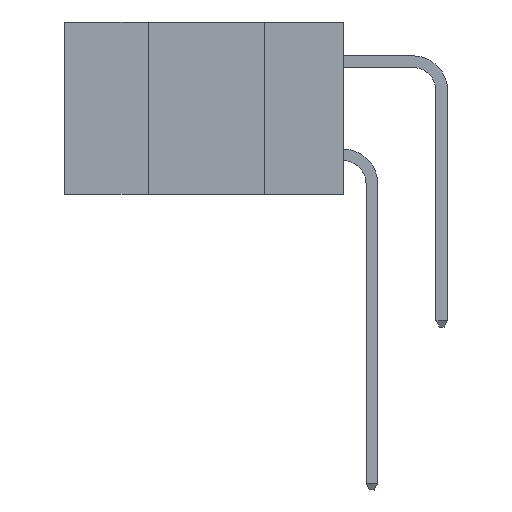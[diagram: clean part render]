
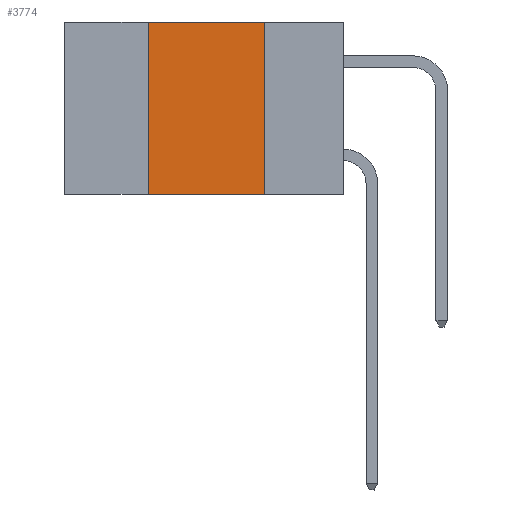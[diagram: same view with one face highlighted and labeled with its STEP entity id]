
A CAD part, left-side view. The second image highlights one B-rep face of the part: STEP entity #3774.
In plain terms, the highlighted planar face has unit normal (-1, 0, 0).
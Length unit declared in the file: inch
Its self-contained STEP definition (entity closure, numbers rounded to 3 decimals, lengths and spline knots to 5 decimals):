
#669 = ORIENTED_EDGE ( 'NONE', *, *, #6722, .T. ) ;
#713 = FACE_OUTER_BOUND ( 'NONE', #1780, .T. ) ;
#848 = CARTESIAN_POINT ( 'NONE',  ( 0., 0.42, 0. ) ) ;
#1388 = DIRECTION ( 'NONE',  ( 0., 0., -1. ) ) ;
#1756 = DIRECTION ( 'NONE',  ( 0., -1., 0. ) ) ;
#1780 = EDGE_LOOP ( 'NONE', ( #10727, #11275, #1974, #669 ) ) ;
#1974 = ORIENTED_EDGE ( 'NONE', *, *, #6973, .F. ) ;
#2211 = VERTEX_POINT ( 'NONE', #6532 ) ;
#2814 = DIRECTION ( 'NONE',  ( 1., 0., 0. ) ) ;
#3587 = AXIS2_PLACEMENT_3D ( 'NONE', #4600, #2814, #1388 ) ;
#3748 = CARTESIAN_POINT ( 'NONE',  ( 0., 0.42, -0.37 ) ) ;
#3774 = ADVANCED_FACE ( 'NONE', ( #713 ), #9079, .F. ) ;
#4600 = CARTESIAN_POINT ( 'NONE',  ( 0., 0.6, 0. ) ) ;
#4678 = CARTESIAN_POINT ( 'NONE',  ( 0., 0.6, 0. ) ) ;
#5889 = CARTESIAN_POINT ( 'NONE',  ( 0., 0.17, -0.37 ) ) ;
#5912 = VECTOR ( 'NONE', #1756, 39.37008 ) ;
#6346 = CARTESIAN_POINT ( 'NONE',  ( 0., 0.6, -0.37 ) ) ;
#6445 = VECTOR ( 'NONE', #9263, 39.37008 ) ;
#6532 = CARTESIAN_POINT ( 'NONE',  ( 0., 0.17, 0. ) ) ;
#6722 = EDGE_CURVE ( 'NONE', #8249, #11709, #11407, .T. ) ;
#6894 = LINE ( 'NONE', #4678, #6445 ) ;
#6973 = EDGE_CURVE ( 'NONE', #8249, #10506, #10831, .T. ) ;
#7071 = EDGE_CURVE ( 'NONE', #2211, #11709, #10114, .T. ) ;
#7792 = VECTOR ( 'NONE', #7807, 39.37008 ) ;
#7807 = DIRECTION ( 'NONE',  ( 0., 0., 1. ) ) ;
#8249 = VERTEX_POINT ( 'NONE', #3748 ) ;
#8517 = EDGE_CURVE ( 'NONE', #10506, #2211, #6894, .T. ) ;
#9079 = PLANE ( 'NONE',  #3587 ) ;
#9263 = DIRECTION ( 'NONE',  ( 0., -1., 0. ) ) ;
#9363 = VECTOR ( 'NONE', #10874, 39.37008 ) ;
#9485 = CARTESIAN_POINT ( 'NONE',  ( 0., 0.42, 0. ) ) ;
#9984 = CARTESIAN_POINT ( 'NONE',  ( 0., 0.17, 0. ) ) ;
#10114 = LINE ( 'NONE', #9984, #9363 ) ;
#10506 = VERTEX_POINT ( 'NONE', #848 ) ;
#10727 = ORIENTED_EDGE ( 'NONE', *, *, #7071, .F. ) ;
#10831 = LINE ( 'NONE', #9485, #7792 ) ;
#10874 = DIRECTION ( 'NONE',  ( 0., 0., -1. ) ) ;
#11275 = ORIENTED_EDGE ( 'NONE', *, *, #8517, .F. ) ;
#11407 = LINE ( 'NONE', #6346, #5912 ) ;
#11709 = VERTEX_POINT ( 'NONE', #5889 ) ;
